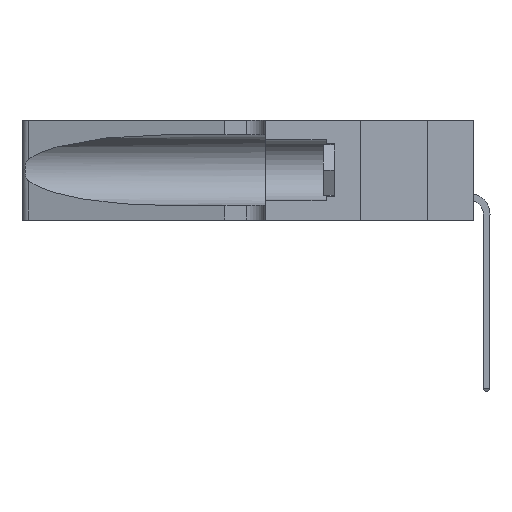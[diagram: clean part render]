
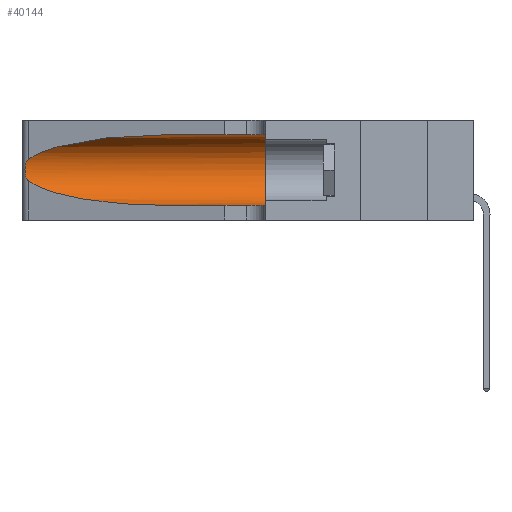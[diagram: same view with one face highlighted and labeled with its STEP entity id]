
A CAD part, left-side view. The second image highlights one B-rep face of the part: STEP entity #40144.
In plain terms, the highlighted cylindrical face has radius 3.308 mm (diameter 6.617 mm), a partial arc.
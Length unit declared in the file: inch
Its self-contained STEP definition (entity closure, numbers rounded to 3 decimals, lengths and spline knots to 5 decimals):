
#138 = EDGE_CURVE ( 'NONE', #1651, #17286, #26085, .T. ) ;
#983 = DIRECTION ( 'NONE',  ( 0., -1., 0. ) ) ;
#1542 = CARTESIAN_POINT ( 'NONE',  ( 0.1305, 0.72297, 0.31525 ) ) ;
#1651 = VERTEX_POINT ( 'NONE', #5748 ) ;
#1831 = EDGE_CURVE ( 'NONE', #33100, #20490, #33073, .T. ) ;
#1881 = ORIENTED_EDGE ( 'NONE', *, *, #26158, .T. ) ;
#2578 = EDGE_LOOP ( 'NONE', ( #33154, #28376, #1881, #28538, #30574, #11864 ) ) ;
#2957 = CARTESIAN_POINT ( 'NONE',  ( 0.25639, 1.23184, 0.21858 ) ) ;
#3075 = VECTOR ( 'NONE', #15977, 39.37008 ) ;
#3219 = CARTESIAN_POINT ( 'NONE',  ( 0.25639, 1.23186, 0.15144 ) ) ;
#4447 = EDGE_CURVE ( 'NONE', #20490, #17286, #7796, .T. ) ;
#4599 = CARTESIAN_POINT ( 'NONE',  ( 0.1305, 0.72297, 0.31525 ) ) ;
#5143 = FACE_OUTER_BOUND ( 'NONE', #2578, .T. ) ;
#5748 = CARTESIAN_POINT ( 'NONE',  ( 0.1305, 0.72297, 0.05475 ) ) ;
#5914 = CARTESIAN_POINT ( 'NONE',  ( 0.25487, 1.22718, 0.22369 ) ) ;
#5993 = CARTESIAN_POINT ( 'NONE',  ( 0.25487, 1.22718, 0.22369 ) ) ;
#6125 = CARTESIAN_POINT ( 'NONE',  ( 0.25854, 1.2359, 0.20912 ) ) ;
#6163 = DIRECTION ( 'NONE',  ( 0., -1., 0. ) ) ;
#7796 = CIRCLE ( 'NONE', #37650, 0.13025 ) ;
#8901 = B_SPLINE_CURVE_WITH_KNOTS ( 'NONE', 3,
 ( #5993, #34306, #2957, #21796, #6125, #28103, #9271, #11813, #33760, #36914, #34665, #3219, #25488, #37696 ),
 .UNSPECIFIED., .F., .F.,
 ( 4, 2, 2, 2, 2, 2, 4 ),
 ( 0., 0.00027, 0.00053, 0.00107, 0.0016, 0.00187, 0.00214 ),
 .UNSPECIFIED. ) ;
#9271 = CARTESIAN_POINT ( 'NONE',  ( 0.26075, 1.23896, 0.19203 ) ) ;
#10814 = CARTESIAN_POINT ( 'NONE',  ( 0.25487, 1.22718, 0.22369 ) ) ;
#11813 = CARTESIAN_POINT ( 'NONE',  ( 0.26075, 1.23896, 0.178 ) ) ;
#11864 = ORIENTED_EDGE ( 'NONE', *, *, #1831, .F. ) ;
#12191 = VERTEX_POINT ( 'NONE', #5914 ) ;
#13279 = EDGE_CURVE ( 'NONE', #33100, #12191, #29532, .T. ) ;
#14273 = CARTESIAN_POINT ( 'NONE',  ( 0.18966, 0.96281, 0.31525 ) ) ;
#14320 = VERTEX_POINT ( 'NONE', #27457 ) ;
#14381 = CARTESIAN_POINT ( 'NONE',  ( 0.1305, 0.35, 0.31525 ) ) ;
#14485 =( BOUNDED_CURVE ( )  B_SPLINE_CURVE ( 3, ( #19242, #22630, #31848, #16116 ),
 .UNSPECIFIED., .F., .F. ) 
 B_SPLINE_CURVE_WITH_KNOTS ( ( 4, 4 ),
 ( 3.44316, 4.71239 ),
 .UNSPECIFIED. ) 
 CURVE ( )  GEOMETRIC_REPRESENTATION_ITEM ( )  RATIONAL_B_SPLINE_CURVE ( ( 1., 0.87, 0.87, 1. ) ) 
 REPRESENTATION_ITEM ( '' )  );
#15511 = DIRECTION ( 'NONE',  ( 0., 0., 1. ) ) ;
#15825 = CARTESIAN_POINT ( 'NONE',  ( 0.1305, 1.61858, 0.05475 ) ) ;
#15977 = DIRECTION ( 'NONE',  ( 0., -1., 0. ) ) ;
#16116 = CARTESIAN_POINT ( 'NONE',  ( 0.1305, 0.72297, 0.05475 ) ) ;
#17286 = VERTEX_POINT ( 'NONE', #36989 ) ;
#17287 = VECTOR ( 'NONE', #6163, 39.37008 ) ;
#17934 = CYLINDRICAL_SURFACE ( 'NONE', #38085, 0.13025 ) ;
#19242 = CARTESIAN_POINT ( 'NONE',  ( 0.25487, 1.22718, 0.14631 ) ) ;
#19874 = CARTESIAN_POINT ( 'NONE',  ( 0.1305, 1.61858, 0.185 ) ) ;
#20490 = VERTEX_POINT ( 'NONE', #14381 ) ;
#21796 = CARTESIAN_POINT ( 'NONE',  ( 0.25787, 1.23484, 0.2124 ) ) ;
#22630 = CARTESIAN_POINT ( 'NONE',  ( 0.2373, 1.15595, 0.08982 ) ) ;
#23163 = CARTESIAN_POINT ( 'NONE',  ( 0.2373, 1.15595, 0.28018 ) ) ;
#25488 = CARTESIAN_POINT ( 'NONE',  ( 0.25555, 1.22993, 0.14849 ) ) ;
#26085 = LINE ( 'NONE', #15825, #17287 ) ;
#26158 = EDGE_CURVE ( 'NONE', #14320, #1651, #14485, .T. ) ;
#26456 = DIRECTION ( 'NONE',  ( 0., 0., -1. ) ) ;
#27457 = CARTESIAN_POINT ( 'NONE',  ( 0.25487, 1.22718, 0.14631 ) ) ;
#28103 = CARTESIAN_POINT ( 'NONE',  ( 0.26018, 1.23835, 0.19895 ) ) ;
#28376 = ORIENTED_EDGE ( 'NONE', *, *, #38571, .T. ) ;
#28538 = ORIENTED_EDGE ( 'NONE', *, *, #138, .T. ) ;
#29532 =( BOUNDED_CURVE ( )  B_SPLINE_CURVE ( 3, ( #1542, #14273, #23163, #10814 ),
 .UNSPECIFIED., .F., .F. ) 
 B_SPLINE_CURVE_WITH_KNOTS ( ( 4, 4 ),
 ( 1.5708, 2.84003 ),
 .UNSPECIFIED. ) 
 CURVE ( )  GEOMETRIC_REPRESENTATION_ITEM ( )  RATIONAL_B_SPLINE_CURVE ( ( 1., 0.87, 0.87, 1. ) ) 
 REPRESENTATION_ITEM ( '' )  );
#30574 = ORIENTED_EDGE ( 'NONE', *, *, #4447, .F. ) ;
#31122 = DIRECTION ( 'NONE',  ( 0., 1., 0. ) ) ;
#31848 = CARTESIAN_POINT ( 'NONE',  ( 0.18966, 0.96281, 0.05475 ) ) ;
#33073 = LINE ( 'NONE', #35002, #3075 ) ;
#33100 = VERTEX_POINT ( 'NONE', #4599 ) ;
#33154 = ORIENTED_EDGE ( 'NONE', *, *, #13279, .T. ) ;
#33760 = CARTESIAN_POINT ( 'NONE',  ( 0.26017, 1.23833, 0.17102 ) ) ;
#34306 = CARTESIAN_POINT ( 'NONE',  ( 0.25555, 1.22994, 0.2215 ) ) ;
#34665 = CARTESIAN_POINT ( 'NONE',  ( 0.25789, 1.23486, 0.15765 ) ) ;
#35002 = CARTESIAN_POINT ( 'NONE',  ( 0.1305, 1.61858, 0.31525 ) ) ;
#36914 = CARTESIAN_POINT ( 'NONE',  ( 0.25856, 1.23593, 0.16098 ) ) ;
#36989 = CARTESIAN_POINT ( 'NONE',  ( 0.1305, 0.35, 0.05475 ) ) ;
#37650 = AXIS2_PLACEMENT_3D ( 'NONE', #37824, #31122, #15511 ) ;
#37696 = CARTESIAN_POINT ( 'NONE',  ( 0.25487, 1.22718, 0.14631 ) ) ;
#37824 = CARTESIAN_POINT ( 'NONE',  ( 0.1305, 0.35, 0.185 ) ) ;
#38085 = AXIS2_PLACEMENT_3D ( 'NONE', #19874, #983, #26456 ) ;
#38571 = EDGE_CURVE ( 'NONE', #12191, #14320, #8901, .T. ) ;
#40144 = ADVANCED_FACE ( 'NONE', ( #5143 ), #17934, .F. ) ;
